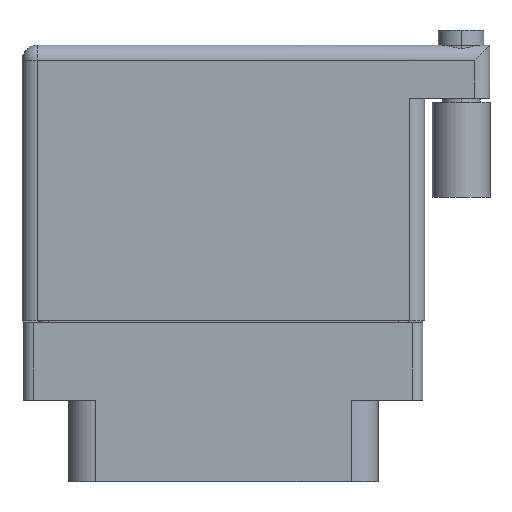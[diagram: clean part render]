
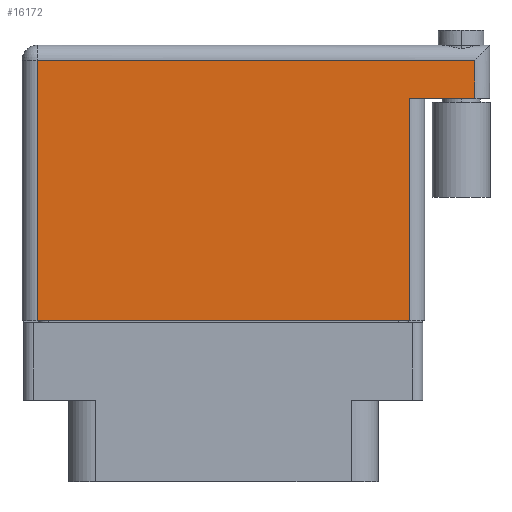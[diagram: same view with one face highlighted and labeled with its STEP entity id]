
A CAD part, front view. The second image highlights one B-rep face of the part: STEP entity #16172.
In plain terms, the highlighted face is planar.
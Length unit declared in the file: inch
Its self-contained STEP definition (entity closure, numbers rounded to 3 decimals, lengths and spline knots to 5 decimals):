
#27 = ORIENTED_EDGE ( 'NONE', *, *, #25424, .T. ) ;
#451 = CARTESIAN_POINT ( 'NONE',  ( 0.6125, -0.1, 0.3575 ) ) ;
#1266 = DIRECTION ( 'NONE',  ( 1., 0., 0. ) ) ;
#2885 = ORIENTED_EDGE ( 'NONE', *, *, #20809, .T. ) ;
#3367 = CARTESIAN_POINT ( 'NONE',  ( -0.6625, 0.756, 0.3575 ) ) ;
#3827 = CARTESIAN_POINT ( 'NONE',  ( -0.6125, -0.1, 0.3575 ) ) ;
#4270 = AXIS2_PLACEMENT_3D ( 'NONE', #18356, #18698, #12517 ) ;
#4301 = EDGE_LOOP ( 'NONE', ( #21766, #19117, #14479, #21885, #27, #2885 ) ) ;
#4910 = VERTEX_POINT ( 'NONE', #3827 ) ;
#5382 = CARTESIAN_POINT ( 'NONE',  ( 0.8765, 0.631, 0.3575 ) ) ;
#5692 = LINE ( 'NONE', #12172, #18378 ) ;
#6583 = DIRECTION ( 'NONE',  ( 0., 1., 0. ) ) ;
#7053 = VECTOR ( 'NONE', #23697, 39.37008 ) ;
#8103 = DIRECTION ( 'NONE',  ( 0., -1., 0. ) ) ;
#8422 = PLANE ( 'NONE',  #4270 ) ;
#8764 = VERTEX_POINT ( 'NONE', #19761 ) ;
#9014 = LINE ( 'NONE', #22964, #17875 ) ;
#9503 = DIRECTION ( 'NONE',  ( -1., 0., 0. ) ) ;
#9802 = LINE ( 'NONE', #5382, #11092 ) ;
#9856 = LINE ( 'NONE', #19863, #7053 ) ;
#11092 = VECTOR ( 'NONE', #9503, 39.37008 ) ;
#12087 = VERTEX_POINT ( 'NONE', #24778 ) ;
#12172 = CARTESIAN_POINT ( 'NONE',  ( -0.6125, -0.1, 0.3575 ) ) ;
#12282 = LINE ( 'NONE', #19663, #17340 ) ;
#12517 = DIRECTION ( 'NONE',  ( -1., 0., 0. ) ) ;
#13541 = DIRECTION ( 'NONE',  ( -1., 0., 0. ) ) ;
#14479 = ORIENTED_EDGE ( 'NONE', *, *, #20599, .F. ) ;
#15972 = EDGE_CURVE ( 'NONE', #4910, #16813, #12282, .T. ) ;
#16172 = ADVANCED_FACE ( 'NONE', ( #23029 ), #8422, .F. ) ;
#16458 = VECTOR ( 'NONE', #13541, 39.37008 ) ;
#16813 = VERTEX_POINT ( 'NONE', #451 ) ;
#17340 = VECTOR ( 'NONE', #1266, 39.37008 ) ;
#17875 = VECTOR ( 'NONE', #6583, 39.37008 ) ;
#18356 = CARTESIAN_POINT ( 'NONE',  ( -0.6625, 0.806, 0.3575 ) ) ;
#18378 = VECTOR ( 'NONE', #8103, 39.37008 ) ;
#18529 = EDGE_CURVE ( 'NONE', #16813, #12087, #9014, .T. ) ;
#18698 = DIRECTION ( 'NONE',  ( 0., 0., -1. ) ) ;
#19117 = ORIENTED_EDGE ( 'NONE', *, *, #18529, .T. ) ;
#19663 = CARTESIAN_POINT ( 'NONE',  ( -0.6625, -0.1, 0.3575 ) ) ;
#19761 = CARTESIAN_POINT ( 'NONE',  ( 0.8265, 0.631, 0.3575 ) ) ;
#19863 = CARTESIAN_POINT ( 'NONE',  ( 0.8265, 0.806, 0.3575 ) ) ;
#20599 = EDGE_CURVE ( 'NONE', #8764, #12087, #9802, .T. ) ;
#20809 = EDGE_CURVE ( 'NONE', #24826, #4910, #5692, .T. ) ;
#21249 = LINE ( 'NONE', #3367, #16458 ) ;
#21271 = VERTEX_POINT ( 'NONE', #23748 ) ;
#21766 = ORIENTED_EDGE ( 'NONE', *, *, #15972, .T. ) ;
#21885 = ORIENTED_EDGE ( 'NONE', *, *, #24190, .T. ) ;
#21992 = CARTESIAN_POINT ( 'NONE',  ( -0.6125, 0.756, 0.3575 ) ) ;
#22964 = CARTESIAN_POINT ( 'NONE',  ( 0.6125, 0.631, 0.3575 ) ) ;
#23029 = FACE_OUTER_BOUND ( 'NONE', #4301, .T. ) ;
#23697 = DIRECTION ( 'NONE',  ( 0., 1., 0. ) ) ;
#23748 = CARTESIAN_POINT ( 'NONE',  ( 0.8265, 0.756, 0.3575 ) ) ;
#24190 = EDGE_CURVE ( 'NONE', #8764, #21271, #9856, .T. ) ;
#24778 = CARTESIAN_POINT ( 'NONE',  ( 0.6125, 0.631, 0.3575 ) ) ;
#24826 = VERTEX_POINT ( 'NONE', #21992 ) ;
#25424 = EDGE_CURVE ( 'NONE', #21271, #24826, #21249, .T. ) ;
